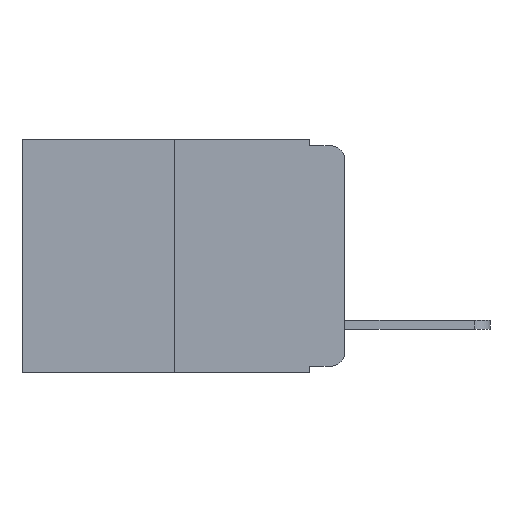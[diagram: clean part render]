
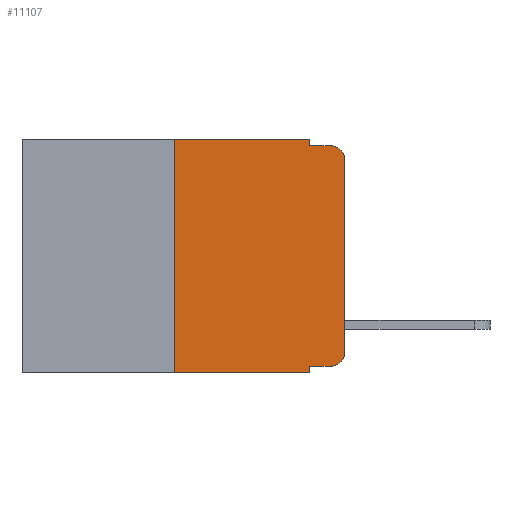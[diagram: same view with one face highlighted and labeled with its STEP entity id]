
A CAD part, left-side view. The second image highlights one B-rep face of the part: STEP entity #11107.
In plain terms, the highlighted planar face has unit normal (-1, 0, 0).
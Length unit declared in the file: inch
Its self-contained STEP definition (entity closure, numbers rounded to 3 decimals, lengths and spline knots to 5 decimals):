
#513 = CIRCLE ( 'NONE', #21577, 0.02 ) ;
#925 = DIRECTION ( 'NONE',  ( 0., 0., 1. ) ) ;
#1558 = CARTESIAN_POINT ( 'NONE',  ( 0., 0.051, 0. ) ) ;
#1762 = DIRECTION ( 'NONE',  ( 0., -1., 0. ) ) ;
#2172 = VERTEX_POINT ( 'NONE', #6991 ) ;
#2487 = VERTEX_POINT ( 'NONE', #4512 ) ;
#3201 = ORIENTED_EDGE ( 'NONE', *, *, #17515, .F. ) ;
#3286 = EDGE_CURVE ( 'NONE', #3675, #18841, #14021, .T. ) ;
#3381 = CIRCLE ( 'NONE', #11606, 0.02 ) ;
#3454 = AXIS2_PLACEMENT_3D ( 'NONE', #14708, #22798, #24680 ) ;
#3507 = VECTOR ( 'NONE', #1762, 39.37008 ) ;
#3675 = VERTEX_POINT ( 'NONE', #6917 ) ;
#3696 = EDGE_CURVE ( 'NONE', #15846, #2487, #513, .T. ) ;
#3942 = LINE ( 'NONE', #5856, #12858 ) ;
#4238 = ORIENTED_EDGE ( 'NONE', *, *, #16377, .T. ) ;
#4512 = CARTESIAN_POINT ( 'NONE',  ( 0., 0.02, -0.01 ) ) ;
#5207 = ORIENTED_EDGE ( 'NONE', *, *, #21451, .F. ) ;
#5300 = VERTEX_POINT ( 'NONE', #12998 ) ;
#5425 = CARTESIAN_POINT ( 'NONE',  ( 0., 0.051, -0.01 ) ) ;
#5856 = CARTESIAN_POINT ( 'NONE',  ( 0., 0.051, -0.333 ) ) ;
#6917 = CARTESIAN_POINT ( 'NONE',  ( 0., 0.25, 0. ) ) ;
#6991 = CARTESIAN_POINT ( 'NONE',  ( 0., 0., -0.313 ) ) ;
#8230 = VECTOR ( 'NONE', #13001, 39.37008 ) ;
#8889 = DIRECTION ( 'NONE',  ( -1., 0., 0. ) ) ;
#8996 = DIRECTION ( 'NONE',  ( -1., 0., 0. ) ) ;
#9039 = VERTEX_POINT ( 'NONE', #16355 ) ;
#9505 = CARTESIAN_POINT ( 'NONE',  ( 0., 0.051, -0.01 ) ) ;
#10018 = LINE ( 'NONE', #9505, #13074 ) ;
#10449 = LINE ( 'NONE', #24442, #15355 ) ;
#10700 = LINE ( 'NONE', #1558, #8230 ) ;
#10768 = DIRECTION ( 'NONE',  ( 0., 0., 1. ) ) ;
#10778 = PLANE ( 'NONE',  #3454 ) ;
#11107 = ADVANCED_FACE ( 'NONE', ( #23377 ), #10778, .F. ) ;
#11205 = CARTESIAN_POINT ( 'NONE',  ( 0., 0.02, -0.313 ) ) ;
#11564 = CARTESIAN_POINT ( 'NONE',  ( 0., 0.473, -0.343 ) ) ;
#11606 = AXIS2_PLACEMENT_3D ( 'NONE', #11205, #8889, #18771 ) ;
#12176 = VERTEX_POINT ( 'NONE', #13523 ) ;
#12199 = EDGE_LOOP ( 'NONE', ( #23969, #17221, #5207, #13500, #23525, #13788, #4238, #3201, #15735, #13518 ) ) ;
#12662 = VERTEX_POINT ( 'NONE', #24484 ) ;
#12832 = EDGE_CURVE ( 'NONE', #12662, #9039, #3942, .T. ) ;
#12858 = VECTOR ( 'NONE', #25405, 39.37008 ) ;
#12889 = CARTESIAN_POINT ( 'NONE',  ( 0., 0.051, 0. ) ) ;
#12998 = CARTESIAN_POINT ( 'NONE',  ( 0., 0.051, -0.343 ) ) ;
#13001 = DIRECTION ( 'NONE',  ( 0., 0., -1. ) ) ;
#13074 = VECTOR ( 'NONE', #21434, 39.37008 ) ;
#13231 = VERTEX_POINT ( 'NONE', #5425 ) ;
#13262 = LINE ( 'NONE', #12889, #16315 ) ;
#13380 = DIRECTION ( 'NONE',  ( 0., -1., 0. ) ) ;
#13500 = ORIENTED_EDGE ( 'NONE', *, *, #20163, .F. ) ;
#13518 = ORIENTED_EDGE ( 'NONE', *, *, #18704, .T. ) ;
#13523 = CARTESIAN_POINT ( 'NONE',  ( 0., 0.25, -0.343 ) ) ;
#13560 = CARTESIAN_POINT ( 'NONE',  ( 0., 0., -0.03 ) ) ;
#13788 = ORIENTED_EDGE ( 'NONE', *, *, #18132, .F. ) ;
#14021 = LINE ( 'NONE', #15418, #18655 ) ;
#14708 = CARTESIAN_POINT ( 'NONE',  ( 0., 0.473, 0. ) ) ;
#15050 = DIRECTION ( 'NONE',  ( 0., 0., -1. ) ) ;
#15355 = VECTOR ( 'NONE', #925, 39.37008 ) ;
#15418 = CARTESIAN_POINT ( 'NONE',  ( 0., 0.473, 0. ) ) ;
#15735 = ORIENTED_EDGE ( 'NONE', *, *, #12832, .T. ) ;
#15846 = VERTEX_POINT ( 'NONE', #13560 ) ;
#16315 = VECTOR ( 'NONE', #21135, 39.37008 ) ;
#16355 = CARTESIAN_POINT ( 'NONE',  ( 0., 0.02, -0.333 ) ) ;
#16377 = EDGE_CURVE ( 'NONE', #12176, #5300, #17967, .T. ) ;
#16712 = CARTESIAN_POINT ( 'NONE',  ( 0., 0.02, -0.03 ) ) ;
#17221 = ORIENTED_EDGE ( 'NONE', *, *, #3696, .T. ) ;
#17515 = EDGE_CURVE ( 'NONE', #12662, #5300, #13262, .T. ) ;
#17967 = LINE ( 'NONE', #11564, #3507 ) ;
#18132 = EDGE_CURVE ( 'NONE', #12176, #3675, #10449, .T. ) ;
#18593 = CARTESIAN_POINT ( 'NONE',  ( 0., 0., 0. ) ) ;
#18655 = VECTOR ( 'NONE', #13380, 39.37008 ) ;
#18704 = EDGE_CURVE ( 'NONE', #9039, #2172, #3381, .T. ) ;
#18771 = DIRECTION ( 'NONE',  ( 0., 0., -1. ) ) ;
#18841 = VERTEX_POINT ( 'NONE', #24999 ) ;
#20163 = EDGE_CURVE ( 'NONE', #18841, #13231, #10700, .T. ) ;
#21135 = DIRECTION ( 'NONE',  ( 0., 0., -1. ) ) ;
#21434 = DIRECTION ( 'NONE',  ( 0., -1., 0. ) ) ;
#21451 = EDGE_CURVE ( 'NONE', #13231, #2487, #10018, .T. ) ;
#21577 = AXIS2_PLACEMENT_3D ( 'NONE', #16712, #8996, #15050 ) ;
#22467 = VECTOR ( 'NONE', #10768, 39.37008 ) ;
#22798 = DIRECTION ( 'NONE',  ( 1., 0., 0. ) ) ;
#23377 = FACE_OUTER_BOUND ( 'NONE', #12199, .T. ) ;
#23525 = ORIENTED_EDGE ( 'NONE', *, *, #3286, .F. ) ;
#23969 = ORIENTED_EDGE ( 'NONE', *, *, #24754, .T. ) ;
#24442 = CARTESIAN_POINT ( 'NONE',  ( 0., 0.25, 0. ) ) ;
#24484 = CARTESIAN_POINT ( 'NONE',  ( 0., 0.051, -0.333 ) ) ;
#24680 = DIRECTION ( 'NONE',  ( 0., 0., -1. ) ) ;
#24754 = EDGE_CURVE ( 'NONE', #2172, #15846, #24899, .T. ) ;
#24899 = LINE ( 'NONE', #18593, #22467 ) ;
#24999 = CARTESIAN_POINT ( 'NONE',  ( 0., 0.051, 0. ) ) ;
#25405 = DIRECTION ( 'NONE',  ( 0., -1., 0. ) ) ;
